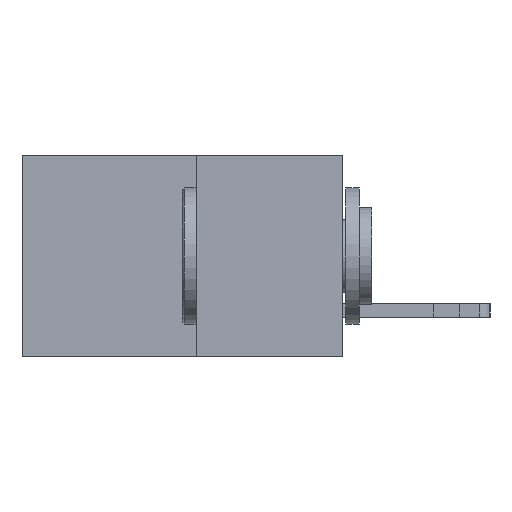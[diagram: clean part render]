
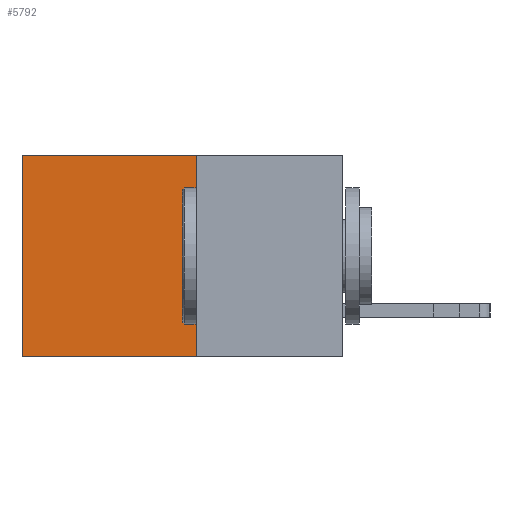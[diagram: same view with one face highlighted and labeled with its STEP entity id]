
A CAD part, left-side view. The second image highlights one B-rep face of the part: STEP entity #5792.
In plain terms, the highlighted planar face has unit normal (-1, 0, 0).
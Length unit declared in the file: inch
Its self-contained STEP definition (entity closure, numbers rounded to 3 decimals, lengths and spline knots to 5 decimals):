
#71 = VERTEX_POINT ( 'NONE', #13016 ) ;
#215 = CARTESIAN_POINT ( 'NONE',  ( 0.277, 0.59, 0. ) ) ;
#327 = VERTEX_POINT ( 'NONE', #9723 ) ;
#805 = VECTOR ( 'NONE', #13354, 39.37008 ) ;
#2176 = VECTOR ( 'NONE', #4986, 39.37008 ) ;
#3395 = VERTEX_POINT ( 'NONE', #215 ) ;
#4920 = VECTOR ( 'NONE', #13843, 39.37008 ) ;
#4952 = CARTESIAN_POINT ( 'NONE',  ( 0.277, 0.27, -0.37 ) ) ;
#4986 = DIRECTION ( 'NONE',  ( 0., 1., 0. ) ) ;
#5593 = ORIENTED_EDGE ( 'NONE', *, *, #8656, .F. ) ;
#5638 = EDGE_CURVE ( 'NONE', #3395, #11307, #15454, .T. ) ;
#5792 = ADVANCED_FACE ( 'NONE', ( #13025 ), #13238, .F. ) ;
#5901 = DIRECTION ( 'NONE',  ( 0., 0., -1. ) ) ;
#6104 = CARTESIAN_POINT ( 'NONE',  ( 0.277, 0.27, -0.37 ) ) ;
#6639 = CARTESIAN_POINT ( 'NONE',  ( 0.277, 0.59, -0.37 ) ) ;
#6761 = EDGE_CURVE ( 'NONE', #327, #3395, #7779, .T. ) ;
#7484 = EDGE_LOOP ( 'NONE', ( #9763, #10216, #5593, #16496 ) ) ;
#7779 = LINE ( 'NONE', #13357, #805 ) ;
#8656 = EDGE_CURVE ( 'NONE', #327, #71, #14331, .T. ) ;
#9723 = CARTESIAN_POINT ( 'NONE',  ( 0.277, 0.27, 0. ) ) ;
#9763 = ORIENTED_EDGE ( 'NONE', *, *, #5638, .T. ) ;
#10216 = ORIENTED_EDGE ( 'NONE', *, *, #12806, .F. ) ;
#10324 = LINE ( 'NONE', #4952, #2176 ) ;
#10419 = DIRECTION ( 'NONE',  ( 0., 0., -1. ) ) ;
#10476 = CARTESIAN_POINT ( 'NONE',  ( 0.277, 0.27, -0.37 ) ) ;
#10665 = DIRECTION ( 'NONE',  ( 1., 0., 0. ) ) ;
#11262 = VECTOR ( 'NONE', #5901, 39.37008 ) ;
#11307 = VERTEX_POINT ( 'NONE', #6639 ) ;
#12188 = AXIS2_PLACEMENT_3D ( 'NONE', #10476, #10665, #10419 ) ;
#12806 = EDGE_CURVE ( 'NONE', #71, #11307, #10324, .T. ) ;
#13016 = CARTESIAN_POINT ( 'NONE',  ( 0.277, 0.27, -0.37 ) ) ;
#13025 = FACE_OUTER_BOUND ( 'NONE', #7484, .T. ) ;
#13238 = PLANE ( 'NONE',  #12188 ) ;
#13354 = DIRECTION ( 'NONE',  ( 0., 1., 0. ) ) ;
#13357 = CARTESIAN_POINT ( 'NONE',  ( 0.277, 0.27, 0. ) ) ;
#13843 = DIRECTION ( 'NONE',  ( 0., 0., -1. ) ) ;
#13861 = CARTESIAN_POINT ( 'NONE',  ( 0.277, 0.59, -0.37 ) ) ;
#14331 = LINE ( 'NONE', #6104, #11262 ) ;
#15454 = LINE ( 'NONE', #13861, #4920 ) ;
#16496 = ORIENTED_EDGE ( 'NONE', *, *, #6761, .T. ) ;
